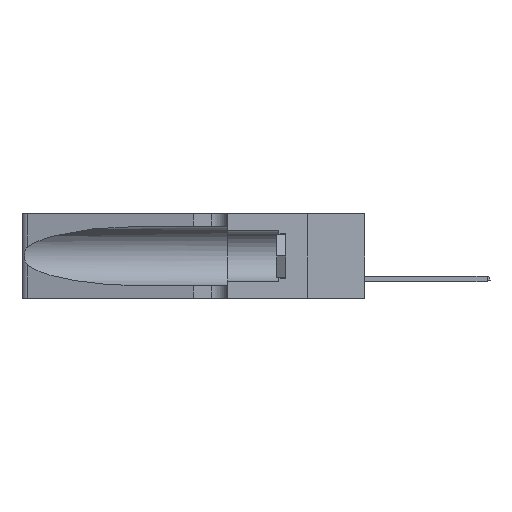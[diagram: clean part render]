
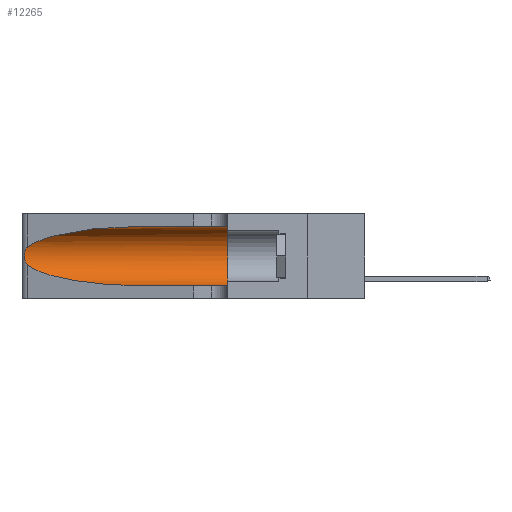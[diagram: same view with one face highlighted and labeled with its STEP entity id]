
A CAD part, left-side view. The second image highlights one B-rep face of the part: STEP entity #12265.
In plain terms, the highlighted cylindrical face has radius 3.308 mm (diameter 6.617 mm), a partial arc.
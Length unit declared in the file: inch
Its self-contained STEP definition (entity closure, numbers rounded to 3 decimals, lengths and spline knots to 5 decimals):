
#1069 = CARTESIAN_POINT ( 'NONE',  ( 0.1305, 0.35, 0.185 ) ) ;
#1154 = CYLINDRICAL_SURFACE ( 'NONE', #47176, 0.13025 ) ;
#1637 = VERTEX_POINT ( 'NONE', #46311 ) ;
#2524 = LINE ( 'NONE', #6164, #40724 ) ;
#3416 = EDGE_CURVE ( 'NONE', #1637, #13462, #33089, .T. ) ;
#4796 = DIRECTION ( 'NONE',  ( 0., -1., 0. ) ) ;
#4799 = EDGE_CURVE ( 'NONE', #12142, #12877, #31613, .T. ) ;
#6164 = CARTESIAN_POINT ( 'NONE',  ( 0.1305, 1.61858, 0.05475 ) ) ;
#6329 =( BOUNDED_CURVE ( )  B_SPLINE_CURVE ( 3, ( #41382, #7660, #21754, #8590 ),
 .UNSPECIFIED., .F., .T. ) 
 B_SPLINE_CURVE_WITH_KNOTS ( ( 4, 4 ),
 ( 1.5708, 2.84003 ),
 .UNSPECIFIED. ) 
 CURVE ( )  GEOMETRIC_REPRESENTATION_ITEM ( )  RATIONAL_B_SPLINE_CURVE ( ( 1., 0.87, 0.87, 1. ) ) 
 REPRESENTATION_ITEM ( '' )  );
#6427 = CARTESIAN_POINT ( 'NONE',  ( 0.26018, 1.23835, 0.19895 ) ) ;
#6762 = CARTESIAN_POINT ( 'NONE',  ( 0.25787, 1.23484, 0.2124 ) ) ;
#7660 = CARTESIAN_POINT ( 'NONE',  ( 0.18966, 0.96281, 0.31525 ) ) ;
#8042 = ORIENTED_EDGE ( 'NONE', *, *, #29078, .T. ) ;
#8350 = VECTOR ( 'NONE', #4796, 39.37008 ) ;
#8590 = CARTESIAN_POINT ( 'NONE',  ( 0.25487, 1.22718, 0.22369 ) ) ;
#8635 = DIRECTION ( 'NONE',  ( 0., 0., -1. ) ) ;
#9229 = EDGE_CURVE ( 'NONE', #13635, #1637, #20648, .T. ) ;
#12142 = VERTEX_POINT ( 'NONE', #13320 ) ;
#12265 = ADVANCED_FACE ( 'NONE', ( #47549 ), #1154, .F. ) ;
#12877 = VERTEX_POINT ( 'NONE', #38866 ) ;
#13320 = CARTESIAN_POINT ( 'NONE',  ( 0.25487, 1.22718, 0.14631 ) ) ;
#13462 = VERTEX_POINT ( 'NONE', #38695 ) ;
#13635 = VERTEX_POINT ( 'NONE', #46048 ) ;
#14530 = AXIS2_PLACEMENT_3D ( 'NONE', #1069, #48379, #24455 ) ;
#14539 = CARTESIAN_POINT ( 'NONE',  ( 0.26075, 1.23896, 0.19203 ) ) ;
#14884 = ORIENTED_EDGE ( 'NONE', *, *, #4799, .T. ) ;
#16236 = CARTESIAN_POINT ( 'NONE',  ( 0.2373, 1.15595, 0.08982 ) ) ;
#16814 = CARTESIAN_POINT ( 'NONE',  ( 0.1305, 1.61858, 0.31525 ) ) ;
#17929 = CARTESIAN_POINT ( 'NONE',  ( 0.26017, 1.23833, 0.17102 ) ) ;
#18500 = CARTESIAN_POINT ( 'NONE',  ( 0.25487, 1.22718, 0.14631 ) ) ;
#20648 = LINE ( 'NONE', #16814, #8350 ) ;
#21062 = CARTESIAN_POINT ( 'NONE',  ( 0.25487, 1.22718, 0.22369 ) ) ;
#21754 = CARTESIAN_POINT ( 'NONE',  ( 0.2373, 1.15595, 0.28018 ) ) ;
#24455 = DIRECTION ( 'NONE',  ( 0., 0., 1. ) ) ;
#26296 = CARTESIAN_POINT ( 'NONE',  ( 0.25856, 1.23593, 0.16098 ) ) ;
#26397 = DIRECTION ( 'NONE',  ( 0., -1., 0. ) ) ;
#29078 = EDGE_CURVE ( 'NONE', #12877, #13462, #2524, .T. ) ;
#30075 = CARTESIAN_POINT ( 'NONE',  ( 0.25854, 1.2359, 0.20912 ) ) ;
#30449 = CARTESIAN_POINT ( 'NONE',  ( 0.25555, 1.22994, 0.2215 ) ) ;
#31149 = ORIENTED_EDGE ( 'NONE', *, *, #48456, .T. ) ;
#31613 =( BOUNDED_CURVE ( )  B_SPLINE_CURVE ( 3, ( #31995, #16236, #43975, #40070 ),
 .UNSPECIFIED., .F., .F. ) 
 B_SPLINE_CURVE_WITH_KNOTS ( ( 4, 4 ),
 ( 3.44316, 4.71239 ),
 .UNSPECIFIED. ) 
 CURVE ( )  GEOMETRIC_REPRESENTATION_ITEM ( )  RATIONAL_B_SPLINE_CURVE ( ( 1., 0.87, 0.87, 1. ) ) 
 REPRESENTATION_ITEM ( '' )  );
#31995 = CARTESIAN_POINT ( 'NONE',  ( 0.25487, 1.22718, 0.14631 ) ) ;
#32426 = CARTESIAN_POINT ( 'NONE',  ( 0.1305, 1.61858, 0.185 ) ) ;
#33089 = CIRCLE ( 'NONE', #14530, 0.13025 ) ;
#33128 = ORIENTED_EDGE ( 'NONE', *, *, #9229, .F. ) ;
#34424 = CARTESIAN_POINT ( 'NONE',  ( 0.25789, 1.23486, 0.15765 ) ) ;
#36896 = VERTEX_POINT ( 'NONE', #21062 ) ;
#37766 = DIRECTION ( 'NONE',  ( 0., -1., 0. ) ) ;
#38023 = CARTESIAN_POINT ( 'NONE',  ( 0.26075, 1.23896, 0.178 ) ) ;
#38376 = CARTESIAN_POINT ( 'NONE',  ( 0.25555, 1.22993, 0.14849 ) ) ;
#38695 = CARTESIAN_POINT ( 'NONE',  ( 0.1305, 0.35, 0.05475 ) ) ;
#38866 = CARTESIAN_POINT ( 'NONE',  ( 0.1305, 0.72297, 0.05475 ) ) ;
#40070 = CARTESIAN_POINT ( 'NONE',  ( 0.1305, 0.72297, 0.05475 ) ) ;
#40724 = VECTOR ( 'NONE', #37766, 39.37008 ) ;
#41382 = CARTESIAN_POINT ( 'NONE',  ( 0.1305, 0.72297, 0.31525 ) ) ;
#41697 = EDGE_LOOP ( 'NONE', ( #43618, #31149, #14884, #8042, #43682, #33128 ) ) ;
#41718 = B_SPLINE_CURVE_WITH_KNOTS ( 'NONE', 3,
 ( #49890, #30449, #50075, #6762, #30075, #6427, #14539, #38023, #17929, #26296, #34424, #42151, #38376, #18500 ),
 .UNSPECIFIED., .F., .F.,
 ( 4, 2, 2, 2, 2, 2, 4 ),
 ( 0., 0.00027, 0.00053, 0.00107, 0.0016, 0.00187, 0.00214 ),
 .UNSPECIFIED. ) ;
#42151 = CARTESIAN_POINT ( 'NONE',  ( 0.25639, 1.23186, 0.15144 ) ) ;
#43618 = ORIENTED_EDGE ( 'NONE', *, *, #45045, .T. ) ;
#43682 = ORIENTED_EDGE ( 'NONE', *, *, #3416, .F. ) ;
#43975 = CARTESIAN_POINT ( 'NONE',  ( 0.18966, 0.96281, 0.05475 ) ) ;
#45045 = EDGE_CURVE ( 'NONE', #13635, #36896, #6329, .T. ) ;
#46048 = CARTESIAN_POINT ( 'NONE',  ( 0.1305, 0.72297, 0.31525 ) ) ;
#46311 = CARTESIAN_POINT ( 'NONE',  ( 0.1305, 0.35, 0.31525 ) ) ;
#47176 = AXIS2_PLACEMENT_3D ( 'NONE', #32426, #26397, #8635 ) ;
#47549 = FACE_OUTER_BOUND ( 'NONE', #41697, .T. ) ;
#48379 = DIRECTION ( 'NONE',  ( 0., 1., 0. ) ) ;
#48456 = EDGE_CURVE ( 'NONE', #36896, #12142, #41718, .T. ) ;
#49890 = CARTESIAN_POINT ( 'NONE',  ( 0.25487, 1.22718, 0.22369 ) ) ;
#50075 = CARTESIAN_POINT ( 'NONE',  ( 0.25639, 1.23184, 0.21858 ) ) ;
